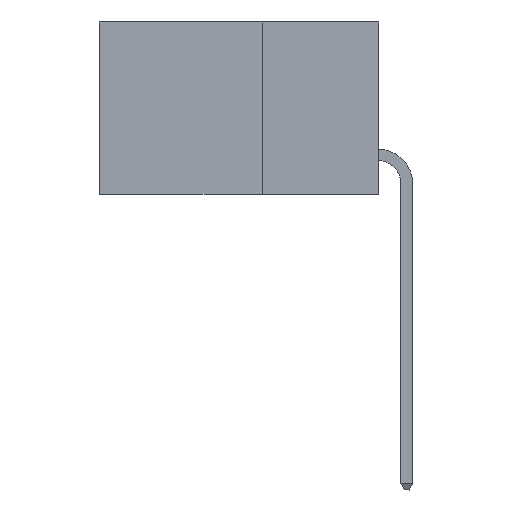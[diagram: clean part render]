
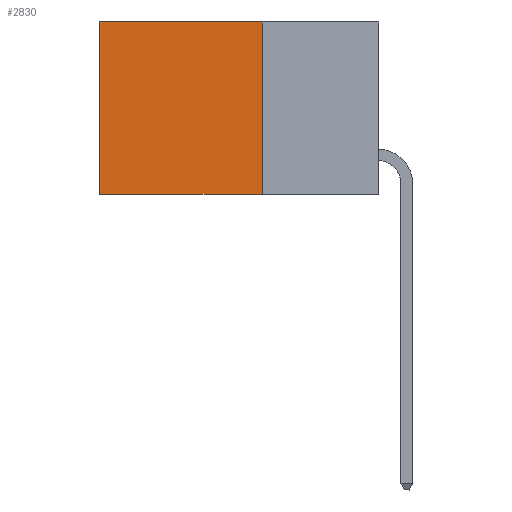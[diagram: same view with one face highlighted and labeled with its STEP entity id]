
A CAD part, left-side view. The second image highlights one B-rep face of the part: STEP entity #2830.
In plain terms, the highlighted planar face has unit normal (-1, 0, 0).
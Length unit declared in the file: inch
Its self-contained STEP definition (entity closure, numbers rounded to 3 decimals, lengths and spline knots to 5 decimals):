
#1069 = CARTESIAN_POINT ( 'NONE',  ( 0.298, 0.25, 0. ) ) ;
#1954 = PLANE ( 'NONE',  #17417 ) ;
#2830 = ADVANCED_FACE ( 'NONE', ( #5884 ), #1954, .F. ) ;
#3410 = VERTEX_POINT ( 'NONE', #5574 ) ;
#3540 = CARTESIAN_POINT ( 'NONE',  ( 0.298, 0.25, -0.37 ) ) ;
#3774 = EDGE_CURVE ( 'NONE', #13793, #3410, #16900, .T. ) ;
#3975 = DIRECTION ( 'NONE',  ( 0., 0., -1. ) ) ;
#4007 = DIRECTION ( 'NONE',  ( 1., 0., 0. ) ) ;
#4732 = LINE ( 'NONE', #14033, #8364 ) ;
#5412 = VECTOR ( 'NONE', #19618, 39.37008 ) ;
#5574 = CARTESIAN_POINT ( 'NONE',  ( 0.298, 0.6, 0. ) ) ;
#5884 = FACE_OUTER_BOUND ( 'NONE', #10471, .T. ) ;
#7526 = EDGE_CURVE ( 'NONE', #3410, #17380, #9050, .T. ) ;
#8364 = VECTOR ( 'NONE', #9526, 39.37008 ) ;
#8459 = ORIENTED_EDGE ( 'NONE', *, *, #16345, .F. ) ;
#8985 = VECTOR ( 'NONE', #16078, 39.37008 ) ;
#9050 = LINE ( 'NONE', #9323, #5412 ) ;
#9323 = CARTESIAN_POINT ( 'NONE',  ( 0.298, 0.6, 0. ) ) ;
#9526 = DIRECTION ( 'NONE',  ( 0., 0., -1. ) ) ;
#9755 = ORIENTED_EDGE ( 'NONE', *, *, #3774, .T. ) ;
#10198 = CARTESIAN_POINT ( 'NONE',  ( 0.298, 0.25, -0.37 ) ) ;
#10471 = EDGE_LOOP ( 'NONE', ( #17994, #8459, #10522, #9755 ) ) ;
#10522 = ORIENTED_EDGE ( 'NONE', *, *, #18551, .F. ) ;
#11516 = VECTOR ( 'NONE', #17624, 39.37008 ) ;
#13793 = VERTEX_POINT ( 'NONE', #18051 ) ;
#14033 = CARTESIAN_POINT ( 'NONE',  ( 0.298, 0.25, 0. ) ) ;
#14482 = CARTESIAN_POINT ( 'NONE',  ( 0.298, 0.25, 0. ) ) ;
#16078 = DIRECTION ( 'NONE',  ( 0., 1., 0. ) ) ;
#16345 = EDGE_CURVE ( 'NONE', #16781, #17380, #19324, .T. ) ;
#16781 = VERTEX_POINT ( 'NONE', #3540 ) ;
#16900 = LINE ( 'NONE', #14482, #8985 ) ;
#17344 = CARTESIAN_POINT ( 'NONE',  ( 0.298, 0.6, -0.37 ) ) ;
#17380 = VERTEX_POINT ( 'NONE', #17344 ) ;
#17417 = AXIS2_PLACEMENT_3D ( 'NONE', #1069, #4007, #3975 ) ;
#17624 = DIRECTION ( 'NONE',  ( 0., 1., 0. ) ) ;
#17994 = ORIENTED_EDGE ( 'NONE', *, *, #7526, .T. ) ;
#18051 = CARTESIAN_POINT ( 'NONE',  ( 0.298, 0.25, 0. ) ) ;
#18551 = EDGE_CURVE ( 'NONE', #13793, #16781, #4732, .T. ) ;
#19324 = LINE ( 'NONE', #10198, #11516 ) ;
#19618 = DIRECTION ( 'NONE',  ( 0., 0., -1. ) ) ;
